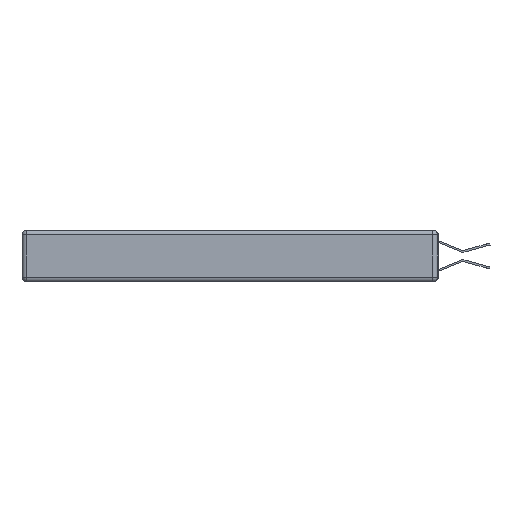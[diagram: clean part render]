
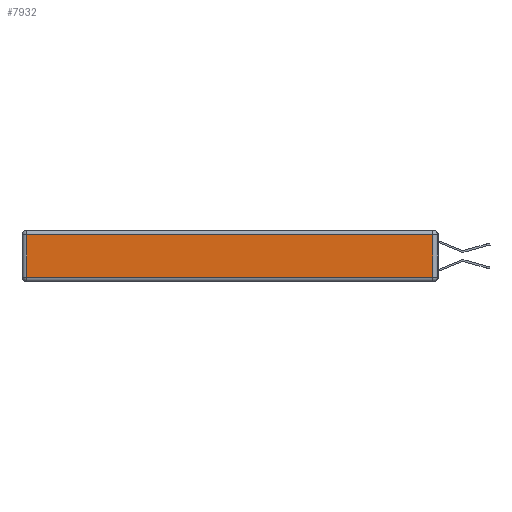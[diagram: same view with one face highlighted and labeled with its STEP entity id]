
A CAD part, left-side view. The second image highlights one B-rep face of the part: STEP entity #7932.
In plain terms, the highlighted planar face has unit normal (-1, 0, 0).
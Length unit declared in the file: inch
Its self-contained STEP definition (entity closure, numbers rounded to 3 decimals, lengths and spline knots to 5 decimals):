
#186 = DIRECTION ( 'NONE',  ( 0., 0., 1. ) ) ;
#253 = EDGE_CURVE ( 'NONE', #15319, #777, #4635, .T. ) ;
#777 = VERTEX_POINT ( 'NONE', #11703 ) ;
#1685 = LINE ( 'NONE', #16578, #7854 ) ;
#2786 = ORIENTED_EDGE ( 'NONE', *, *, #253, .T. ) ;
#2923 = CARTESIAN_POINT ( 'NONE',  ( 0., 0., -0.343 ) ) ;
#3021 = FACE_OUTER_BOUND ( 'NONE', #11485, .T. ) ;
#4113 = EDGE_CURVE ( 'NONE', #12074, #4994, #17271, .T. ) ;
#4461 = DIRECTION ( 'NONE',  ( -1., 0., 0. ) ) ;
#4616 = VECTOR ( 'NONE', #15696, 39.37008 ) ;
#4635 = LINE ( 'NONE', #12883, #4616 ) ;
#4994 = VERTEX_POINT ( 'NONE', #17562 ) ;
#5645 = PLANE ( 'NONE',  #6660 ) ;
#6560 = LINE ( 'NONE', #13699, #9283 ) ;
#6660 = AXIS2_PLACEMENT_3D ( 'NONE', #2923, #4461, #186 ) ;
#7487 = CARTESIAN_POINT ( 'NONE',  ( 0., 2.72, -0.343 ) ) ;
#7742 = VECTOR ( 'NONE', #14367, 39.37008 ) ;
#7854 = VECTOR ( 'NONE', #15390, 39.37008 ) ;
#7932 = ADVANCED_FACE ( 'NONE', ( #3021 ), #5645, .T. ) ;
#9056 = ORIENTED_EDGE ( 'NONE', *, *, #4113, .T. ) ;
#9283 = VECTOR ( 'NONE', #9508, 39.37008 ) ;
#9508 = DIRECTION ( 'NONE',  ( 0., -1., 0. ) ) ;
#11485 = EDGE_LOOP ( 'NONE', ( #15733, #2786, #14000, #9056 ) ) ;
#11703 = CARTESIAN_POINT ( 'NONE',  ( 0., 0.03, -0.03 ) ) ;
#12074 = VERTEX_POINT ( 'NONE', #12391 ) ;
#12115 = EDGE_CURVE ( 'NONE', #777, #12074, #1685, .T. ) ;
#12391 = CARTESIAN_POINT ( 'NONE',  ( 0., 2.72, -0.03 ) ) ;
#12883 = CARTESIAN_POINT ( 'NONE',  ( 0., 0.03, -0.343 ) ) ;
#13699 = CARTESIAN_POINT ( 'NONE',  ( 0., 0., -0.313 ) ) ;
#14000 = ORIENTED_EDGE ( 'NONE', *, *, #12115, .T. ) ;
#14367 = DIRECTION ( 'NONE',  ( 0., 0., -1. ) ) ;
#15319 = VERTEX_POINT ( 'NONE', #15454 ) ;
#15390 = DIRECTION ( 'NONE',  ( 0., 1., 0. ) ) ;
#15454 = CARTESIAN_POINT ( 'NONE',  ( 0., 0.03, -0.313 ) ) ;
#15696 = DIRECTION ( 'NONE',  ( 0., 0., 1. ) ) ;
#15733 = ORIENTED_EDGE ( 'NONE', *, *, #16959, .T. ) ;
#16578 = CARTESIAN_POINT ( 'NONE',  ( 0., 2.75, -0.03 ) ) ;
#16959 = EDGE_CURVE ( 'NONE', #4994, #15319, #6560, .T. ) ;
#17271 = LINE ( 'NONE', #7487, #7742 ) ;
#17562 = CARTESIAN_POINT ( 'NONE',  ( 0., 2.72, -0.313 ) ) ;
